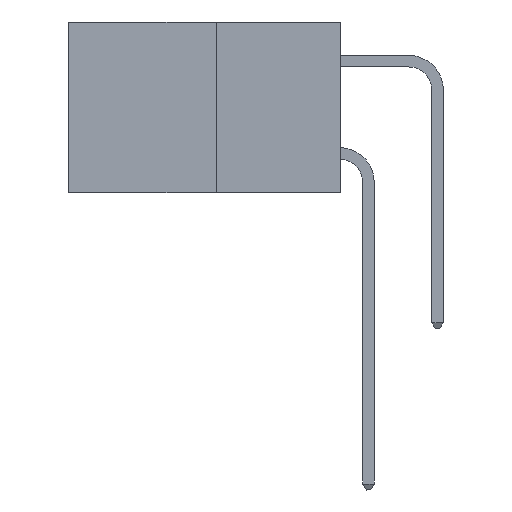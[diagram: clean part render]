
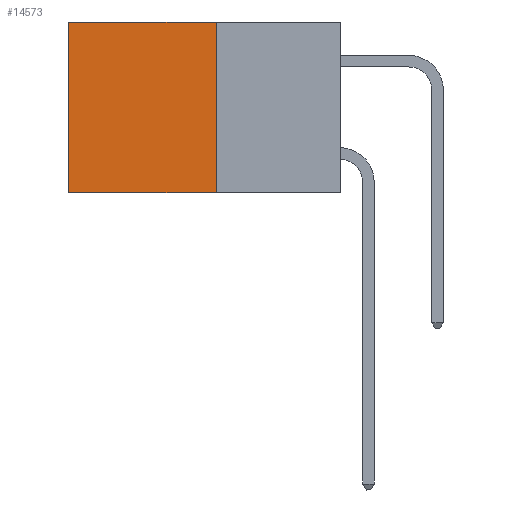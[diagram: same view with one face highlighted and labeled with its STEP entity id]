
A CAD part, left-side view. The second image highlights one B-rep face of the part: STEP entity #14573.
In plain terms, the highlighted planar face has unit normal (-1, 0, 0).
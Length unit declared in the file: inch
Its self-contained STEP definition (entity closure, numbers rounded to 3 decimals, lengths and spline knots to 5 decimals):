
#50 = PLANE ( 'NONE',  #23122 ) ;
#2470 = CARTESIAN_POINT ( 'NONE',  ( 0.277, 0.59, -0.37 ) ) ;
#3067 = EDGE_CURVE ( 'NONE', #20882, #31720, #11773, .T. ) ;
#3219 = LINE ( 'NONE', #2470, #31505 ) ;
#5259 = ORIENTED_EDGE ( 'NONE', *, *, #3067, .F. ) ;
#5656 = CARTESIAN_POINT ( 'NONE',  ( 0.277, 0.27, -0.37 ) ) ;
#5729 = CARTESIAN_POINT ( 'NONE',  ( 0.277, 0.59, 0. ) ) ;
#6099 = VERTEX_POINT ( 'NONE', #11989 ) ;
#8727 = CARTESIAN_POINT ( 'NONE',  ( 0.277, 0.27, -0.37 ) ) ;
#9940 = VECTOR ( 'NONE', #13303, 39.37008 ) ;
#9997 = ORIENTED_EDGE ( 'NONE', *, *, #22888, .F. ) ;
#10017 = DIRECTION ( 'NONE',  ( 0., 0., -1. ) ) ;
#10139 = CARTESIAN_POINT ( 'NONE',  ( 0.277, 0.27, -0.37 ) ) ;
#10156 = CARTESIAN_POINT ( 'NONE',  ( 0.277, 0.27, -0.37 ) ) ;
#11773 = LINE ( 'NONE', #10139, #31136 ) ;
#11989 = CARTESIAN_POINT ( 'NONE',  ( 0.277, 0.59, -0.37 ) ) ;
#12006 = FACE_OUTER_BOUND ( 'NONE', #19499, .T. ) ;
#12781 = LINE ( 'NONE', #10156, #24325 ) ;
#12799 = DIRECTION ( 'NONE',  ( 0., 1., 0. ) ) ;
#13303 = DIRECTION ( 'NONE',  ( 0., 1., 0. ) ) ;
#13770 = DIRECTION ( 'NONE',  ( 0., 0., -1. ) ) ;
#14441 = EDGE_CURVE ( 'NONE', #20882, #21105, #22350, .T. ) ;
#14573 = ADVANCED_FACE ( 'NONE', ( #12006 ), #50, .F. ) ;
#19499 = EDGE_LOOP ( 'NONE', ( #24323, #9997, #5259, #21232 ) ) ;
#20882 = VERTEX_POINT ( 'NONE', #28825 ) ;
#21105 = VERTEX_POINT ( 'NONE', #5729 ) ;
#21232 = ORIENTED_EDGE ( 'NONE', *, *, #14441, .T. ) ;
#21271 = DIRECTION ( 'NONE',  ( 0., 0., -1. ) ) ;
#22350 = LINE ( 'NONE', #29089, #9940 ) ;
#22888 = EDGE_CURVE ( 'NONE', #31720, #6099, #12781, .T. ) ;
#23122 = AXIS2_PLACEMENT_3D ( 'NONE', #5656, #29539, #13770 ) ;
#24323 = ORIENTED_EDGE ( 'NONE', *, *, #25300, .T. ) ;
#24325 = VECTOR ( 'NONE', #12799, 39.37008 ) ;
#25300 = EDGE_CURVE ( 'NONE', #21105, #6099, #3219, .T. ) ;
#28825 = CARTESIAN_POINT ( 'NONE',  ( 0.277, 0.27, 0. ) ) ;
#29089 = CARTESIAN_POINT ( 'NONE',  ( 0.277, 0.27, 0. ) ) ;
#29539 = DIRECTION ( 'NONE',  ( 1., 0., 0. ) ) ;
#31136 = VECTOR ( 'NONE', #10017, 39.37008 ) ;
#31505 = VECTOR ( 'NONE', #21271, 39.37008 ) ;
#31720 = VERTEX_POINT ( 'NONE', #8727 ) ;
